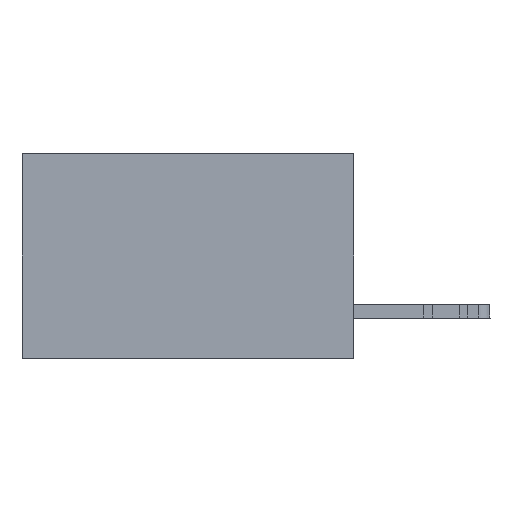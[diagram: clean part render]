
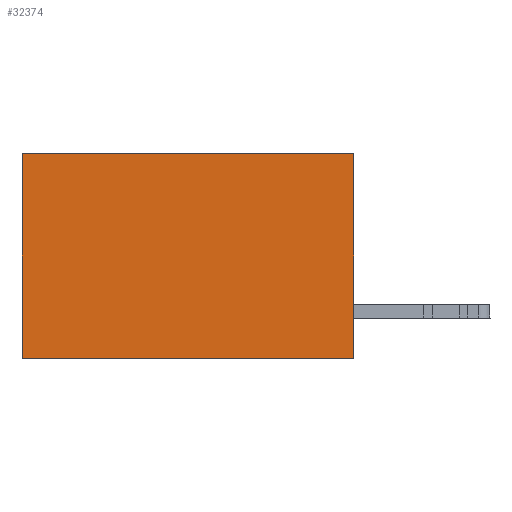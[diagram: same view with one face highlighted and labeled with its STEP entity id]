
A CAD part, left-side view. The second image highlights one B-rep face of the part: STEP entity #32374.
In plain terms, the highlighted planar face has unit normal (-1, 0, 0).
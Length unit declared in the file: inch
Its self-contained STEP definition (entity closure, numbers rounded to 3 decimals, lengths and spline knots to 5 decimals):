
#1793 = CARTESIAN_POINT ( 'NONE',  ( 0.2875, 0., 0. ) ) ;
#2830 = LINE ( 'NONE', #3518, #37764 ) ;
#3518 = CARTESIAN_POINT ( 'NONE',  ( 0.2875, 0., 0. ) ) ;
#5592 = DIRECTION ( 'NONE',  ( 1., 0., 0. ) ) ;
#6108 = EDGE_LOOP ( 'NONE', ( #20227, #33405, #21548, #27151 ) ) ;
#6336 = LINE ( 'NONE', #1793, #39074 ) ;
#6499 = DIRECTION ( 'NONE',  ( 0., 1., 0. ) ) ;
#6788 = VECTOR ( 'NONE', #17052, 39.37008 ) ;
#7164 = DIRECTION ( 'NONE',  ( 0., 0., -1. ) ) ;
#9039 = LINE ( 'NONE', #35191, #46361 ) ;
#9702 = DIRECTION ( 'NONE',  ( 0., 1., 0. ) ) ;
#14328 = VERTEX_POINT ( 'NONE', #42716 ) ;
#14387 = VERTEX_POINT ( 'NONE', #15492 ) ;
#15492 = CARTESIAN_POINT ( 'NONE',  ( 0.2875, 0.6, -0.37 ) ) ;
#17052 = DIRECTION ( 'NONE',  ( 0., 0., -1. ) ) ;
#18009 = LINE ( 'NONE', #38684, #6788 ) ;
#19750 = DIRECTION ( 'NONE',  ( 0., 0., -1. ) ) ;
#20227 = ORIENTED_EDGE ( 'NONE', *, *, #28955, .T. ) ;
#21548 = ORIENTED_EDGE ( 'NONE', *, *, #42740, .F. ) ;
#23917 = AXIS2_PLACEMENT_3D ( 'NONE', #30630, #5592, #19750 ) ;
#23978 = EDGE_CURVE ( 'NONE', #14328, #14387, #9039, .T. ) ;
#24063 = PLANE ( 'NONE',  #23917 ) ;
#24931 = FACE_OUTER_BOUND ( 'NONE', #6108, .T. ) ;
#27151 = ORIENTED_EDGE ( 'NONE', *, *, #32356, .T. ) ;
#28955 = EDGE_CURVE ( 'NONE', #31405, #14387, #18009, .T. ) ;
#30630 = CARTESIAN_POINT ( 'NONE',  ( 0.2875, 0., 0. ) ) ;
#31405 = VERTEX_POINT ( 'NONE', #43105 ) ;
#32356 = EDGE_CURVE ( 'NONE', #38135, #31405, #6336, .T. ) ;
#32374 = ADVANCED_FACE ( 'NONE', ( #24931 ), #24063, .F. ) ;
#33405 = ORIENTED_EDGE ( 'NONE', *, *, #23978, .F. ) ;
#34896 = CARTESIAN_POINT ( 'NONE',  ( 0.2875, 0., 0. ) ) ;
#35191 = CARTESIAN_POINT ( 'NONE',  ( 0.2875, 0., -0.37 ) ) ;
#37764 = VECTOR ( 'NONE', #7164, 39.37008 ) ;
#38135 = VERTEX_POINT ( 'NONE', #34896 ) ;
#38684 = CARTESIAN_POINT ( 'NONE',  ( 0.2875, 0.6, 0. ) ) ;
#39074 = VECTOR ( 'NONE', #9702, 39.37008 ) ;
#42716 = CARTESIAN_POINT ( 'NONE',  ( 0.2875, 0., -0.37 ) ) ;
#42740 = EDGE_CURVE ( 'NONE', #38135, #14328, #2830, .T. ) ;
#43105 = CARTESIAN_POINT ( 'NONE',  ( 0.2875, 0.6, 0. ) ) ;
#46361 = VECTOR ( 'NONE', #6499, 39.37008 ) ;
